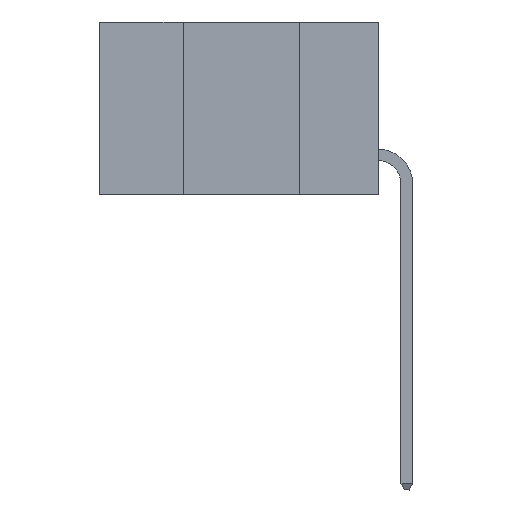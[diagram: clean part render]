
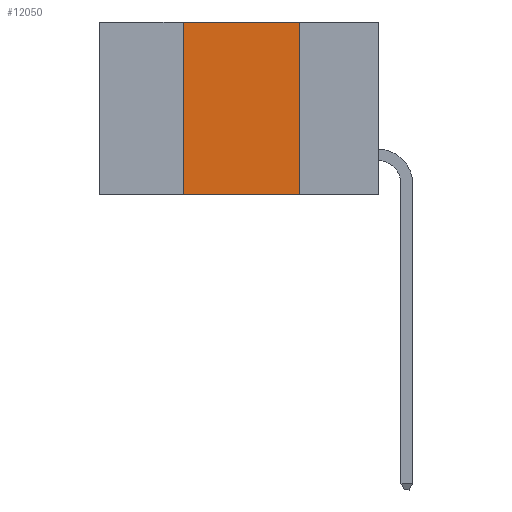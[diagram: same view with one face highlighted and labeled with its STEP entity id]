
A CAD part, left-side view. The second image highlights one B-rep face of the part: STEP entity #12050.
In plain terms, the highlighted planar face has unit normal (-1, 0, 0).
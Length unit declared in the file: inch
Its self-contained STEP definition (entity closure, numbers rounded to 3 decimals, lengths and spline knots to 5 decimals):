
#156 = VECTOR ( 'NONE', #21156, 39.37008 ) ;
#1078 = DIRECTION ( 'NONE',  ( 0., -1., 0. ) ) ;
#1604 = CARTESIAN_POINT ( 'NONE',  ( 0., 0.17, -0.37 ) ) ;
#1914 = CARTESIAN_POINT ( 'NONE',  ( 0., 0.17, 0. ) ) ;
#2102 = LINE ( 'NONE', #11319, #7985 ) ;
#2128 = EDGE_CURVE ( 'NONE', #6656, #12715, #2102, .T. ) ;
#3001 = ORIENTED_EDGE ( 'NONE', *, *, #9565, .F. ) ;
#3216 = DIRECTION ( 'NONE',  ( 1., 0., 0. ) ) ;
#3983 = DIRECTION ( 'NONE',  ( 0., -1., 0. ) ) ;
#6656 = VERTEX_POINT ( 'NONE', #1914 ) ;
#7331 = CARTESIAN_POINT ( 'NONE',  ( 0., 0.42, 0. ) ) ;
#7985 = VECTOR ( 'NONE', #9721, 39.37008 ) ;
#8412 = DIRECTION ( 'NONE',  ( 0., 0., -1. ) ) ;
#8821 = CARTESIAN_POINT ( 'NONE',  ( 0., 0.42, -0.37 ) ) ;
#9565 = EDGE_CURVE ( 'NONE', #20756, #6656, #15495, .T. ) ;
#9721 = DIRECTION ( 'NONE',  ( 0., 0., -1. ) ) ;
#11319 = CARTESIAN_POINT ( 'NONE',  ( 0., 0.17, -0.37 ) ) ;
#12050 = ADVANCED_FACE ( 'NONE', ( #23478 ), #14367, .F. ) ;
#12715 = VERTEX_POINT ( 'NONE', #1604 ) ;
#13757 = LINE ( 'NONE', #15205, #156 ) ;
#14243 = CARTESIAN_POINT ( 'NONE',  ( 0., 0.6, 0. ) ) ;
#14367 = PLANE ( 'NONE',  #23704 ) ;
#15205 = CARTESIAN_POINT ( 'NONE',  ( 0., 0.42, -0.37 ) ) ;
#15252 = LINE ( 'NONE', #18884, #17865 ) ;
#15328 = VERTEX_POINT ( 'NONE', #8821 ) ;
#15495 = LINE ( 'NONE', #19624, #21675 ) ;
#16979 = EDGE_CURVE ( 'NONE', #15328, #20756, #13757, .T. ) ;
#17865 = VECTOR ( 'NONE', #3983, 39.37008 ) ;
#18477 = ORIENTED_EDGE ( 'NONE', *, *, #23133, .T. ) ;
#18884 = CARTESIAN_POINT ( 'NONE',  ( 0., 0.6, -0.37 ) ) ;
#19624 = CARTESIAN_POINT ( 'NONE',  ( 0., 0.6, 0. ) ) ;
#20756 = VERTEX_POINT ( 'NONE', #7331 ) ;
#20947 = ORIENTED_EDGE ( 'NONE', *, *, #16979, .F. ) ;
#21156 = DIRECTION ( 'NONE',  ( 0., 0., 1. ) ) ;
#21675 = VECTOR ( 'NONE', #1078, 39.37008 ) ;
#23133 = EDGE_CURVE ( 'NONE', #15328, #12715, #15252, .T. ) ;
#23478 = FACE_OUTER_BOUND ( 'NONE', #23699, .T. ) ;
#23495 = ORIENTED_EDGE ( 'NONE', *, *, #2128, .F. ) ;
#23699 = EDGE_LOOP ( 'NONE', ( #23495, #3001, #20947, #18477 ) ) ;
#23704 = AXIS2_PLACEMENT_3D ( 'NONE', #14243, #3216, #8412 ) ;
